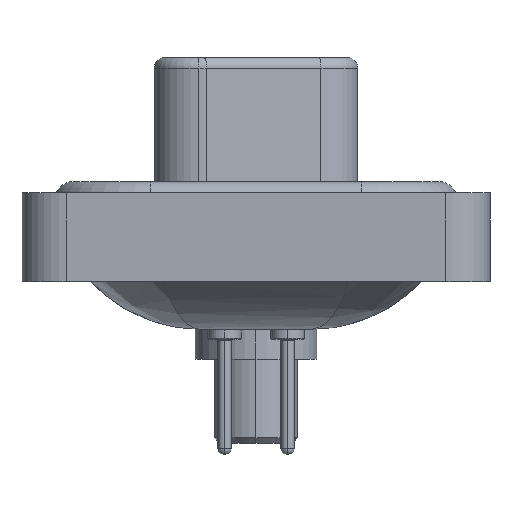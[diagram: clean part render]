
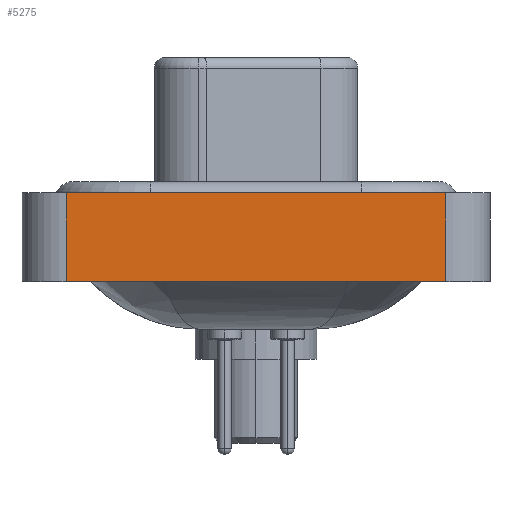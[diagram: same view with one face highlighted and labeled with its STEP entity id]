
A CAD part, left-side view. The second image highlights one B-rep face of the part: STEP entity #5275.
In plain terms, the highlighted planar face has unit normal (-1, 0, 0).
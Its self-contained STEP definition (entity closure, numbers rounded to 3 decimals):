
#134 = CARTESIAN_POINT ( 'NONE',  ( -7.25, -8.55, -3.6 ) ) ;
#342 = VERTEX_POINT ( 'NONE', #10115 ) ;
#879 = LINE ( 'NONE', #7735, #12481 ) ;
#949 = EDGE_CURVE ( 'NONE', #7612, #3534, #7628, .T. ) ;
#1029 = CARTESIAN_POINT ( 'NONE',  ( -7.25, -8.55, -3.6 ) ) ;
#1972 = CARTESIAN_POINT ( 'NONE',  ( -7.25, -8.55, -3.6 ) ) ;
#3002 = EDGE_LOOP ( 'NONE', ( #16274, #12992, #7369, #14250 ) ) ;
#3534 = VERTEX_POINT ( 'NONE', #10063 ) ;
#4497 = LINE ( 'NONE', #134, #11594 ) ;
#5275 = ADVANCED_FACE ( 'NONE', ( #10321 ), #10052, .T. ) ;
#5835 = DIRECTION ( 'NONE',  ( 0., 0., 1. ) ) ;
#6082 = CARTESIAN_POINT ( 'NONE',  ( -7.25, 8.55, 0.4 ) ) ;
#7369 = ORIENTED_EDGE ( 'NONE', *, *, #15988, .F. ) ;
#7612 = VERTEX_POINT ( 'NONE', #13209 ) ;
#7628 = LINE ( 'NONE', #1029, #8892 ) ;
#7735 = CARTESIAN_POINT ( 'NONE',  ( -7.25, 8.55, -3.6 ) ) ;
#8892 = VECTOR ( 'NONE', #12989, 1000. ) ;
#9782 = CARTESIAN_POINT ( 'NONE',  ( -7.25, -8.55, 0.4 ) ) ;
#10052 = PLANE ( 'NONE',  #11075 ) ;
#10063 = CARTESIAN_POINT ( 'NONE',  ( -7.25, -8.55, -3.6 ) ) ;
#10115 = CARTESIAN_POINT ( 'NONE',  ( -7.25, -8.55, 0.4 ) ) ;
#10321 = FACE_OUTER_BOUND ( 'NONE', #3002, .T. ) ;
#11075 = AXIS2_PLACEMENT_3D ( 'NONE', #1972, #12855, #16927 ) ;
#11179 = VERTEX_POINT ( 'NONE', #6082 ) ;
#11487 = EDGE_CURVE ( 'NONE', #11179, #342, #16483, .T. ) ;
#11594 = VECTOR ( 'NONE', #5835, 1000. ) ;
#12481 = VECTOR ( 'NONE', #15659, 1000. ) ;
#12855 = DIRECTION ( 'NONE',  ( -1., 0., 0. ) ) ;
#12989 = DIRECTION ( 'NONE',  ( 0., -1., 0. ) ) ;
#12992 = ORIENTED_EDGE ( 'NONE', *, *, #11487, .F. ) ;
#13209 = CARTESIAN_POINT ( 'NONE',  ( -7.25, 8.55, -3.6 ) ) ;
#13885 = EDGE_CURVE ( 'NONE', #3534, #342, #4497, .T. ) ;
#14250 = ORIENTED_EDGE ( 'NONE', *, *, #949, .T. ) ;
#15141 = DIRECTION ( 'NONE',  ( 0., -1., 0. ) ) ;
#15659 = DIRECTION ( 'NONE',  ( 0., 0., 1. ) ) ;
#15988 = EDGE_CURVE ( 'NONE', #7612, #11179, #879, .T. ) ;
#16274 = ORIENTED_EDGE ( 'NONE', *, *, #13885, .T. ) ;
#16483 = LINE ( 'NONE', #9782, #16638 ) ;
#16638 = VECTOR ( 'NONE', #15141, 1000. ) ;
#16927 = DIRECTION ( 'NONE',  ( 0., 0., 1. ) ) ;
